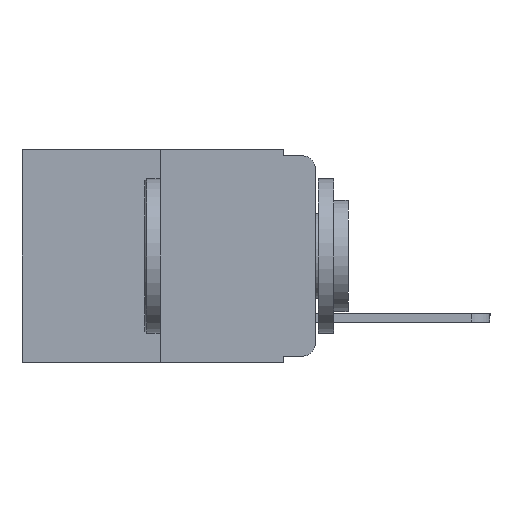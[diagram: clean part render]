
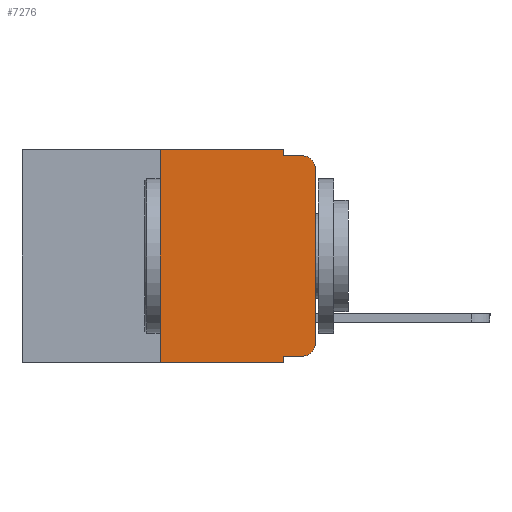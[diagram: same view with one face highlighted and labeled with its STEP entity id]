
A CAD part, left-side view. The second image highlights one B-rep face of the part: STEP entity #7276.
In plain terms, the highlighted planar face has unit normal (-1, 0, 0).
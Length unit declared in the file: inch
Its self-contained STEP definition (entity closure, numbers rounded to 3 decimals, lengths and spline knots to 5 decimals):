
#33 = CIRCLE ( 'NONE', #9415, 0.02 ) ;
#199 = CARTESIAN_POINT ( 'NONE',  ( 0., 0.25, 0. ) ) ;
#300 = CARTESIAN_POINT ( 'NONE',  ( 0., 0., -0.313 ) ) ;
#450 = DIRECTION ( 'NONE',  ( 0., 0., -1. ) ) ;
#519 = DIRECTION ( 'NONE',  ( -1., 0., 0. ) ) ;
#607 = CARTESIAN_POINT ( 'NONE',  ( 0., 0.473, 0. ) ) ;
#677 = VECTOR ( 'NONE', #4427, 39.37008 ) ;
#781 = CARTESIAN_POINT ( 'NONE',  ( 0., 0.02, -0.01 ) ) ;
#873 = VERTEX_POINT ( 'NONE', #3969 ) ;
#967 = EDGE_CURVE ( 'NONE', #7973, #1097, #1226, .T. ) ;
#1097 = VERTEX_POINT ( 'NONE', #300 ) ;
#1115 = LINE ( 'NONE', #9319, #3559 ) ;
#1226 = CIRCLE ( 'NONE', #8407, 0.02 ) ;
#1307 = CARTESIAN_POINT ( 'NONE',  ( 0., 0.051, -0.01 ) ) ;
#1323 = VERTEX_POINT ( 'NONE', #10395 ) ;
#1806 = DIRECTION ( 'NONE',  ( 0., 0., -1. ) ) ;
#1824 = CARTESIAN_POINT ( 'NONE',  ( 0., 0.051, -0.01 ) ) ;
#1912 = VERTEX_POINT ( 'NONE', #8717 ) ;
#1940 = VECTOR ( 'NONE', #9425, 39.37008 ) ;
#2036 = CARTESIAN_POINT ( 'NONE',  ( 0., 0.02, -0.333 ) ) ;
#2053 = VERTEX_POINT ( 'NONE', #6184 ) ;
#2068 = CARTESIAN_POINT ( 'NONE',  ( 0., 0.02, -0.03 ) ) ;
#3244 = EDGE_CURVE ( 'NONE', #6375, #873, #5735, .T. ) ;
#3415 = VECTOR ( 'NONE', #11034, 39.37008 ) ;
#3534 = EDGE_CURVE ( 'NONE', #1912, #8448, #33, .T. ) ;
#3559 = VECTOR ( 'NONE', #3743, 39.37008 ) ;
#3694 = VERTEX_POINT ( 'NONE', #1824 ) ;
#3743 = DIRECTION ( 'NONE',  ( 0., 0., -1. ) ) ;
#3969 = CARTESIAN_POINT ( 'NONE',  ( 0., 0.051, -0.343 ) ) ;
#4048 = EDGE_LOOP ( 'NONE', ( #4280, #4313, #4354, #4510, #4565, #4579, #4645, #4727, #4841, #4951 ) ) ;
#4280 = ORIENTED_EDGE ( 'NONE', *, *, #10485, .T. ) ;
#4313 = ORIENTED_EDGE ( 'NONE', *, *, #3534, .T. ) ;
#4354 = ORIENTED_EDGE ( 'NONE', *, *, #12041, .F. ) ;
#4427 = DIRECTION ( 'NONE',  ( 0., 0., -1. ) ) ;
#4432 = EDGE_CURVE ( 'NONE', #2053, #7973, #10043, .T. ) ;
#4467 = DIRECTION ( 'NONE',  ( 0., -1., 0. ) ) ;
#4490 = AXIS2_PLACEMENT_3D ( 'NONE', #607, #7641, #1806 ) ;
#4510 = ORIENTED_EDGE ( 'NONE', *, *, #9402, .F. ) ;
#4565 = ORIENTED_EDGE ( 'NONE', *, *, #7115, .F. ) ;
#4579 = ORIENTED_EDGE ( 'NONE', *, *, #8795, .F. ) ;
#4645 = ORIENTED_EDGE ( 'NONE', *, *, #3244, .T. ) ;
#4727 = ORIENTED_EDGE ( 'NONE', *, *, #7623, .F. ) ;
#4773 = PLANE ( 'NONE',  #4490 ) ;
#4815 = CARTESIAN_POINT ( 'NONE',  ( 0., 0., 0. ) ) ;
#4841 = ORIENTED_EDGE ( 'NONE', *, *, #4432, .T. ) ;
#4951 = ORIENTED_EDGE ( 'NONE', *, *, #967, .T. ) ;
#5325 = CARTESIAN_POINT ( 'NONE',  ( 0., 0.051, -0.333 ) ) ;
#5495 = FACE_OUTER_BOUND ( 'NONE', #4048, .T. ) ;
#5735 = LINE ( 'NONE', #6195, #10377 ) ;
#6133 = DIRECTION ( 'NONE',  ( 0., -1., 0. ) ) ;
#6181 = VECTOR ( 'NONE', #7197, 39.37008 ) ;
#6184 = CARTESIAN_POINT ( 'NONE',  ( 0., 0.051, -0.333 ) ) ;
#6195 = CARTESIAN_POINT ( 'NONE',  ( 0., 0.473, -0.343 ) ) ;
#6375 = VERTEX_POINT ( 'NONE', #11393 ) ;
#7115 = EDGE_CURVE ( 'NONE', #7976, #1323, #11987, .T. ) ;
#7122 = LINE ( 'NONE', #4815, #1940 ) ;
#7197 = DIRECTION ( 'NONE',  ( 0., -1., 0. ) ) ;
#7276 = ADVANCED_FACE ( 'NONE', ( #5495 ), #4773, .F. ) ;
#7623 = EDGE_CURVE ( 'NONE', #2053, #873, #12297, .T. ) ;
#7624 = VECTOR ( 'NONE', #4467, 39.37008 ) ;
#7641 = DIRECTION ( 'NONE',  ( 1., 0., 0. ) ) ;
#7973 = VERTEX_POINT ( 'NONE', #2036 ) ;
#7976 = VERTEX_POINT ( 'NONE', #9618 ) ;
#8047 = CARTESIAN_POINT ( 'NONE',  ( 0., 0.473, 0. ) ) ;
#8407 = AXIS2_PLACEMENT_3D ( 'NONE', #8736, #11883, #11095 ) ;
#8439 = LINE ( 'NONE', #199, #3415 ) ;
#8448 = VERTEX_POINT ( 'NONE', #781 ) ;
#8508 = DIRECTION ( 'NONE',  ( 0., -1., 0. ) ) ;
#8717 = CARTESIAN_POINT ( 'NONE',  ( 0., 0., -0.03 ) ) ;
#8736 = CARTESIAN_POINT ( 'NONE',  ( 0., 0.02, -0.313 ) ) ;
#8795 = EDGE_CURVE ( 'NONE', #6375, #7976, #8439, .T. ) ;
#9319 = CARTESIAN_POINT ( 'NONE',  ( 0., 0.051, 0. ) ) ;
#9365 = VECTOR ( 'NONE', #8508, 39.37008 ) ;
#9402 = EDGE_CURVE ( 'NONE', #1323, #3694, #1115, .T. ) ;
#9415 = AXIS2_PLACEMENT_3D ( 'NONE', #2068, #519, #450 ) ;
#9425 = DIRECTION ( 'NONE',  ( 0., 0., 1. ) ) ;
#9618 = CARTESIAN_POINT ( 'NONE',  ( 0., 0.25, 0. ) ) ;
#10016 = CARTESIAN_POINT ( 'NONE',  ( 0., 0.051, 0. ) ) ;
#10043 = LINE ( 'NONE', #5325, #7624 ) ;
#10377 = VECTOR ( 'NONE', #6133, 39.37008 ) ;
#10395 = CARTESIAN_POINT ( 'NONE',  ( 0., 0.051, 0. ) ) ;
#10485 = EDGE_CURVE ( 'NONE', #1097, #1912, #7122, .T. ) ;
#11034 = DIRECTION ( 'NONE',  ( 0., 0., 1. ) ) ;
#11095 = DIRECTION ( 'NONE',  ( 0., 0., -1. ) ) ;
#11234 = LINE ( 'NONE', #1307, #6181 ) ;
#11393 = CARTESIAN_POINT ( 'NONE',  ( 0., 0.25, -0.343 ) ) ;
#11883 = DIRECTION ( 'NONE',  ( -1., 0., 0. ) ) ;
#11987 = LINE ( 'NONE', #8047, #9365 ) ;
#12041 = EDGE_CURVE ( 'NONE', #3694, #8448, #11234, .T. ) ;
#12297 = LINE ( 'NONE', #10016, #677 ) ;
